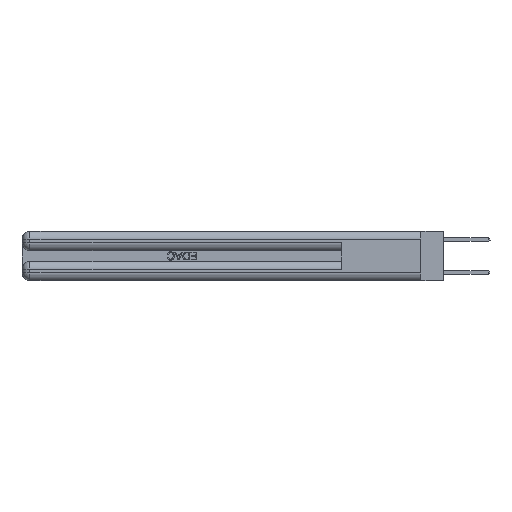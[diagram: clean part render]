
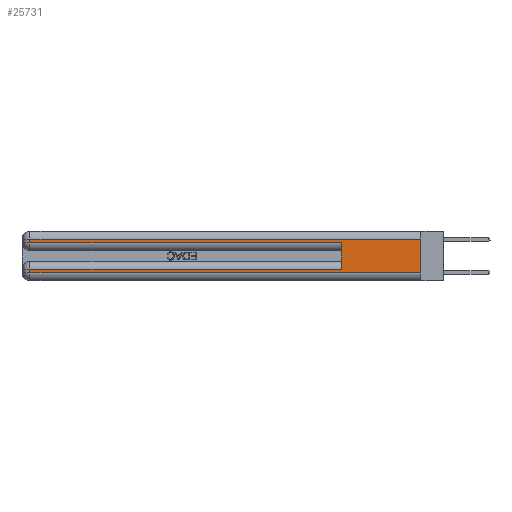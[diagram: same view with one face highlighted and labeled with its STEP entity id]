
A CAD part, left-side view. The second image highlights one B-rep face of the part: STEP entity #25731.
In plain terms, the highlighted planar face has unit normal (-1, 0, 0).
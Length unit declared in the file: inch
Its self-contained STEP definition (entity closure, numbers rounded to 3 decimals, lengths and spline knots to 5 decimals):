
#109 = ORIENTED_EDGE ( 'NONE', *, *, #5749, .T. ) ;
#1070 = DIRECTION ( 'NONE',  ( 0., 1., 0. ) ) ;
#1193 = EDGE_CURVE ( 'NONE', #29854, #26077, #32472, .T. ) ;
#1241 = EDGE_CURVE ( 'NONE', #7717, #26077, #26689, .T. ) ;
#1681 = DIRECTION ( 'NONE',  ( 0., 0., -1. ) ) ;
#1697 = CARTESIAN_POINT ( 'NONE',  ( 0., 0., 0.285 ) ) ;
#1945 = LINE ( 'NONE', #12970, #35542 ) ;
#2239 = DIRECTION ( 'NONE',  ( 0., 0., 1. ) ) ;
#2323 = ORIENTED_EDGE ( 'NONE', *, *, #11877, .T. ) ;
#2963 = CARTESIAN_POINT ( 'NONE',  ( 0., 0., 0.31 ) ) ;
#3563 = VERTEX_POINT ( 'NONE', #9168 ) ;
#3920 = LINE ( 'NONE', #20577, #9920 ) ;
#4034 = CARTESIAN_POINT ( 'NONE',  ( 0., 0., 0.37 ) ) ;
#4414 = DIRECTION ( 'NONE',  ( 0., -1., 0. ) ) ;
#5058 = EDGE_CURVE ( 'NONE', #16476, #17957, #30486, .T. ) ;
#5749 = EDGE_CURVE ( 'NONE', #3563, #7717, #24417, .T. ) ;
#6277 = ORIENTED_EDGE ( 'NONE', *, *, #25513, .T. ) ;
#6433 = DIRECTION ( 'NONE',  ( 0., -1., 0. ) ) ;
#7120 = EDGE_LOOP ( 'NONE', ( #30364, #16921, #109, #20980, #22580, #6277, #19481, #2323 ) ) ;
#7717 = VERTEX_POINT ( 'NONE', #15350 ) ;
#9168 = CARTESIAN_POINT ( 'NONE',  ( 0., 2.94, 0.31 ) ) ;
#9636 = VECTOR ( 'NONE', #19079, 39.37008 ) ;
#9920 = VECTOR ( 'NONE', #6433, 39.37008 ) ;
#10744 = CARTESIAN_POINT ( 'NONE',  ( 0., 0., 0.085 ) ) ;
#11877 = EDGE_CURVE ( 'NONE', #17957, #28735, #3920, .T. ) ;
#12970 = CARTESIAN_POINT ( 'NONE',  ( 0., 0., 0.37 ) ) ;
#13031 = CARTESIAN_POINT ( 'NONE',  ( 0., 0., 0.06 ) ) ;
#14813 = LINE ( 'NONE', #25885, #27290 ) ;
#15350 = CARTESIAN_POINT ( 'NONE',  ( 0., 2.94, 0.285 ) ) ;
#15706 = VECTOR ( 'NONE', #4414, 39.37008 ) ;
#16476 = VERTEX_POINT ( 'NONE', #26961 ) ;
#16921 = ORIENTED_EDGE ( 'NONE', *, *, #33168, .T. ) ;
#17957 = VERTEX_POINT ( 'NONE', #22776 ) ;
#19079 = DIRECTION ( 'NONE',  ( 0., 1., 0. ) ) ;
#19481 = ORIENTED_EDGE ( 'NONE', *, *, #5058, .T. ) ;
#19503 = EDGE_CURVE ( 'NONE', #29252, #28735, #1945, .T. ) ;
#19976 = DIRECTION ( 'NONE',  ( 0., 0., -1. ) ) ;
#20577 = CARTESIAN_POINT ( 'NONE',  ( 0., 0., 0.06 ) ) ;
#20954 = DIRECTION ( 'NONE',  ( 0., 0., -1. ) ) ;
#20980 = ORIENTED_EDGE ( 'NONE', *, *, #1241, .T. ) ;
#22580 = ORIENTED_EDGE ( 'NONE', *, *, #1193, .F. ) ;
#22776 = CARTESIAN_POINT ( 'NONE',  ( 0., 2.94, 0.06 ) ) ;
#23556 = AXIS2_PLACEMENT_3D ( 'NONE', #4034, #25957, #1681 ) ;
#24417 = LINE ( 'NONE', #32406, #31835 ) ;
#25227 = CARTESIAN_POINT ( 'NONE',  ( 0., 2.94, 0.37 ) ) ;
#25513 = EDGE_CURVE ( 'NONE', #29854, #16476, #34360, .T. ) ;
#25731 = ADVANCED_FACE ( 'NONE', ( #29017 ), #31747, .F. ) ;
#25885 = CARTESIAN_POINT ( 'NONE',  ( 0., 0., 0.31 ) ) ;
#25957 = DIRECTION ( 'NONE',  ( 1., 0., 0. ) ) ;
#26077 = VERTEX_POINT ( 'NONE', #33913 ) ;
#26689 = LINE ( 'NONE', #1697, #15706 ) ;
#26961 = CARTESIAN_POINT ( 'NONE',  ( 0., 2.94, 0.085 ) ) ;
#27290 = VECTOR ( 'NONE', #1070, 39.37008 ) ;
#28735 = VERTEX_POINT ( 'NONE', #13031 ) ;
#29017 = FACE_OUTER_BOUND ( 'NONE', #7120, .T. ) ;
#29252 = VERTEX_POINT ( 'NONE', #2963 ) ;
#29854 = VERTEX_POINT ( 'NONE', #33721 ) ;
#29867 = DIRECTION ( 'NONE',  ( 0., 0., -1. ) ) ;
#30364 = ORIENTED_EDGE ( 'NONE', *, *, #19503, .F. ) ;
#30486 = LINE ( 'NONE', #25227, #32453 ) ;
#31747 = PLANE ( 'NONE',  #23556 ) ;
#31835 = VECTOR ( 'NONE', #29867, 39.37008 ) ;
#32406 = CARTESIAN_POINT ( 'NONE',  ( 0., 2.94, 0.37 ) ) ;
#32453 = VECTOR ( 'NONE', #19976, 39.37008 ) ;
#32472 = LINE ( 'NONE', #32660, #32496 ) ;
#32496 = VECTOR ( 'NONE', #2239, 39.37008 ) ;
#32660 = CARTESIAN_POINT ( 'NONE',  ( 0., 0.6, 0.145 ) ) ;
#33168 = EDGE_CURVE ( 'NONE', #29252, #3563, #14813, .T. ) ;
#33721 = CARTESIAN_POINT ( 'NONE',  ( 0., 0.6, 0.085 ) ) ;
#33913 = CARTESIAN_POINT ( 'NONE',  ( 0., 0.6, 0.285 ) ) ;
#34360 = LINE ( 'NONE', #10744, #9636 ) ;
#35542 = VECTOR ( 'NONE', #20954, 39.37008 ) ;
